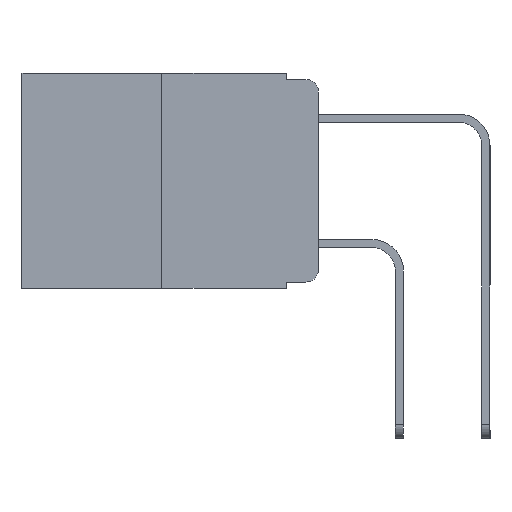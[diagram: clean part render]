
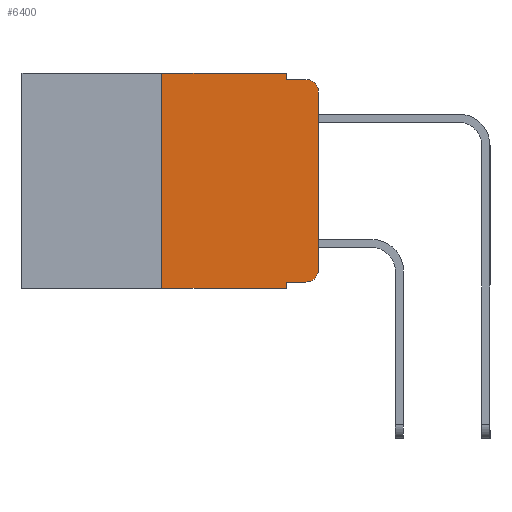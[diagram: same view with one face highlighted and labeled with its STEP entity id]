
A CAD part, left-side view. The second image highlights one B-rep face of the part: STEP entity #6400.
In plain terms, the highlighted planar face has unit normal (-1, 0, 0).
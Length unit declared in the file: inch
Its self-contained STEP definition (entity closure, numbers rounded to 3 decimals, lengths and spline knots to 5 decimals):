
#91 = ORIENTED_EDGE ( 'NONE', *, *, #8495, .F. ) ;
#160 = VECTOR ( 'NONE', #2012, 39.37008 ) ;
#411 = EDGE_CURVE ( 'NONE', #10627, #6241, #13288, .T. ) ;
#492 = CARTESIAN_POINT ( 'NONE',  ( 0., 0.051, -0.333 ) ) ;
#728 = VERTEX_POINT ( 'NONE', #9043 ) ;
#999 = DIRECTION ( 'NONE',  ( 0., -1., 0. ) ) ;
#1080 = EDGE_LOOP ( 'NONE', ( #2057, #7792, #13228, #8461, #91, #3795, #1192, #10083, #12777, #2228 ) ) ;
#1192 = ORIENTED_EDGE ( 'NONE', *, *, #11676, .T. ) ;
#1526 = VECTOR ( 'NONE', #9432, 39.37008 ) ;
#1558 = CARTESIAN_POINT ( 'NONE',  ( 0., 0.02, -0.03 ) ) ;
#1599 = VERTEX_POINT ( 'NONE', #4831 ) ;
#1743 = DIRECTION ( 'NONE',  ( 0., 0., -1. ) ) ;
#1828 = VERTEX_POINT ( 'NONE', #6394 ) ;
#1881 = DIRECTION ( 'NONE',  ( -1., 0., 0. ) ) ;
#1962 = EDGE_CURVE ( 'NONE', #728, #11466, #7287, .T. ) ;
#2012 = DIRECTION ( 'NONE',  ( 0., 0., 1. ) ) ;
#2057 = ORIENTED_EDGE ( 'NONE', *, *, #7036, .T. ) ;
#2228 = ORIENTED_EDGE ( 'NONE', *, *, #6507, .T. ) ;
#2674 = DIRECTION ( 'NONE',  ( 0., 0., -1. ) ) ;
#3029 = CARTESIAN_POINT ( 'NONE',  ( 0., 0.051, -0.333 ) ) ;
#3070 = CARTESIAN_POINT ( 'NONE',  ( 0., 0.051, 0. ) ) ;
#3384 = EDGE_CURVE ( 'NONE', #3444, #1828, #7249, .T. ) ;
#3444 = VERTEX_POINT ( 'NONE', #492 ) ;
#3445 = EDGE_CURVE ( 'NONE', #11466, #1599, #3743, .T. ) ;
#3645 = DIRECTION ( 'NONE',  ( 0., 0., -1. ) ) ;
#3682 = LINE ( 'NONE', #5436, #6541 ) ;
#3743 = LINE ( 'NONE', #5979, #6277 ) ;
#3795 = ORIENTED_EDGE ( 'NONE', *, *, #411, .F. ) ;
#4831 = CARTESIAN_POINT ( 'NONE',  ( 0., 0.02, -0.01 ) ) ;
#5200 = LINE ( 'NONE', #8093, #13103 ) ;
#5436 = CARTESIAN_POINT ( 'NONE',  ( 0., 0.473, 0. ) ) ;
#5568 = CIRCLE ( 'NONE', #10259, 0.02 ) ;
#5625 = EDGE_CURVE ( 'NONE', #7580, #1599, #5568, .T. ) ;
#5911 = CARTESIAN_POINT ( 'NONE',  ( 0., 0.473, -0.343 ) ) ;
#5979 = CARTESIAN_POINT ( 'NONE',  ( 0., 0.051, -0.01 ) ) ;
#5993 = AXIS2_PLACEMENT_3D ( 'NONE', #7132, #8207, #1743 ) ;
#6093 = VECTOR ( 'NONE', #6944, 39.37008 ) ;
#6095 = PLANE ( 'NONE',  #5993 ) ;
#6241 = VERTEX_POINT ( 'NONE', #10965 ) ;
#6277 = VECTOR ( 'NONE', #11179, 39.37008 ) ;
#6394 = CARTESIAN_POINT ( 'NONE',  ( 0., 0.051, -0.343 ) ) ;
#6400 = ADVANCED_FACE ( 'NONE', ( #8193 ), #6095, .F. ) ;
#6507 = EDGE_CURVE ( 'NONE', #8633, #10516, #6539, .T. ) ;
#6539 = CIRCLE ( 'NONE', #8104, 0.02 ) ;
#6541 = VECTOR ( 'NONE', #999, 39.37008 ) ;
#6944 = DIRECTION ( 'NONE',  ( 0., -1., 0. ) ) ;
#7036 = EDGE_CURVE ( 'NONE', #10516, #7580, #5200, .T. ) ;
#7132 = CARTESIAN_POINT ( 'NONE',  ( 0., 0.473, 0. ) ) ;
#7201 = CARTESIAN_POINT ( 'NONE',  ( 0., 0., -0.313 ) ) ;
#7249 = LINE ( 'NONE', #3070, #12722 ) ;
#7287 = LINE ( 'NONE', #8691, #1526 ) ;
#7355 = CARTESIAN_POINT ( 'NONE',  ( 0., 0.25, 0. ) ) ;
#7580 = VERTEX_POINT ( 'NONE', #7932 ) ;
#7792 = ORIENTED_EDGE ( 'NONE', *, *, #5625, .T. ) ;
#7858 = EDGE_CURVE ( 'NONE', #3444, #8633, #11593, .T. ) ;
#7932 = CARTESIAN_POINT ( 'NONE',  ( 0., 0., -0.03 ) ) ;
#8093 = CARTESIAN_POINT ( 'NONE',  ( 0., 0., 0. ) ) ;
#8104 = AXIS2_PLACEMENT_3D ( 'NONE', #8338, #1881, #9383 ) ;
#8193 = FACE_OUTER_BOUND ( 'NONE', #1080, .T. ) ;
#8207 = DIRECTION ( 'NONE',  ( 1., 0., 0. ) ) ;
#8338 = CARTESIAN_POINT ( 'NONE',  ( 0., 0.02, -0.313 ) ) ;
#8353 = DIRECTION ( 'NONE',  ( 0., -1., 0. ) ) ;
#8461 = ORIENTED_EDGE ( 'NONE', *, *, #1962, .F. ) ;
#8495 = EDGE_CURVE ( 'NONE', #6241, #728, #3682, .T. ) ;
#8633 = VERTEX_POINT ( 'NONE', #9842 ) ;
#8691 = CARTESIAN_POINT ( 'NONE',  ( 0., 0.051, 0. ) ) ;
#8858 = VECTOR ( 'NONE', #8353, 39.37008 ) ;
#8879 = CARTESIAN_POINT ( 'NONE',  ( 0., 0.051, -0.01 ) ) ;
#9043 = CARTESIAN_POINT ( 'NONE',  ( 0., 0.051, 0. ) ) ;
#9083 = DIRECTION ( 'NONE',  ( -1., 0., 0. ) ) ;
#9150 = DIRECTION ( 'NONE',  ( 0., 0., 1. ) ) ;
#9207 = LINE ( 'NONE', #5911, #6093 ) ;
#9383 = DIRECTION ( 'NONE',  ( 0., 0., -1. ) ) ;
#9432 = DIRECTION ( 'NONE',  ( 0., 0., -1. ) ) ;
#9842 = CARTESIAN_POINT ( 'NONE',  ( 0., 0.02, -0.333 ) ) ;
#10083 = ORIENTED_EDGE ( 'NONE', *, *, #3384, .F. ) ;
#10259 = AXIS2_PLACEMENT_3D ( 'NONE', #1558, #9083, #2674 ) ;
#10516 = VERTEX_POINT ( 'NONE', #7201 ) ;
#10627 = VERTEX_POINT ( 'NONE', #12521 ) ;
#10965 = CARTESIAN_POINT ( 'NONE',  ( 0., 0.25, 0. ) ) ;
#11179 = DIRECTION ( 'NONE',  ( 0., -1., 0. ) ) ;
#11466 = VERTEX_POINT ( 'NONE', #8879 ) ;
#11593 = LINE ( 'NONE', #3029, #8858 ) ;
#11676 = EDGE_CURVE ( 'NONE', #10627, #1828, #9207, .T. ) ;
#12521 = CARTESIAN_POINT ( 'NONE',  ( 0., 0.25, -0.343 ) ) ;
#12722 = VECTOR ( 'NONE', #3645, 39.37008 ) ;
#12777 = ORIENTED_EDGE ( 'NONE', *, *, #7858, .T. ) ;
#13103 = VECTOR ( 'NONE', #9150, 39.37008 ) ;
#13228 = ORIENTED_EDGE ( 'NONE', *, *, #3445, .F. ) ;
#13288 = LINE ( 'NONE', #7355, #160 ) ;
